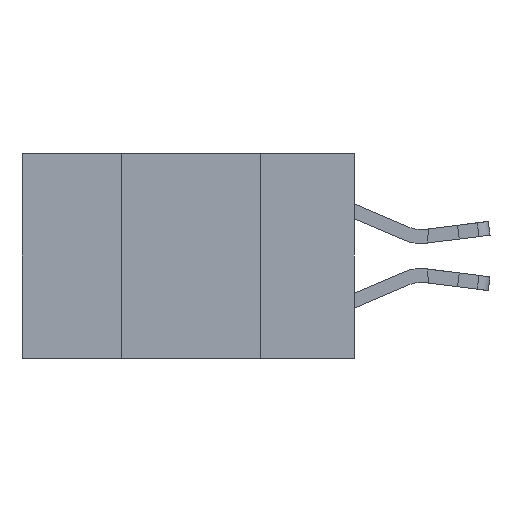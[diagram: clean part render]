
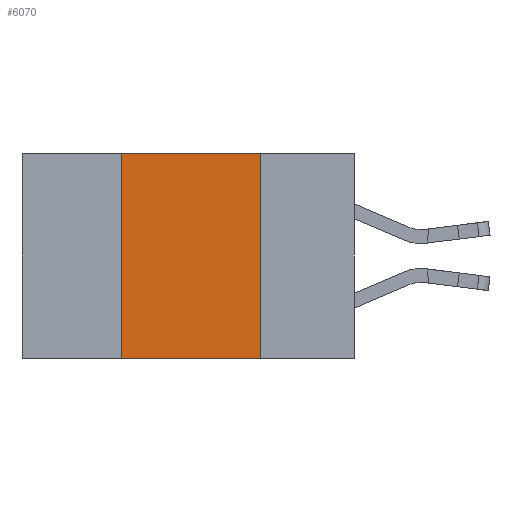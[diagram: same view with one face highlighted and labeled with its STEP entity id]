
A CAD part, left-side view. The second image highlights one B-rep face of the part: STEP entity #6070.
In plain terms, the highlighted planar face has unit normal (-1, 0, 0).
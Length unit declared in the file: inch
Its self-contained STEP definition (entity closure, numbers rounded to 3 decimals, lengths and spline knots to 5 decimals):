
#163 = CARTESIAN_POINT ( 'NONE',  ( 0., 0.17, 0. ) ) ;
#285 = LINE ( 'NONE', #12719, #1492 ) ;
#478 = EDGE_CURVE ( 'NONE', #17541, #1094, #5635, .T. ) ;
#940 = ORIENTED_EDGE ( 'NONE', *, *, #6986, .T. ) ;
#1094 = VERTEX_POINT ( 'NONE', #5809 ) ;
#1492 = VECTOR ( 'NONE', #6743, 39.37008 ) ;
#2147 = PLANE ( 'NONE',  #19913 ) ;
#2264 = ORIENTED_EDGE ( 'NONE', *, *, #478, .F. ) ;
#2501 = DIRECTION ( 'NONE',  ( 0., 0., -1. ) ) ;
#3178 = VECTOR ( 'NONE', #17279, 39.37008 ) ;
#5108 = ORIENTED_EDGE ( 'NONE', *, *, #9924, .F. ) ;
#5505 = CARTESIAN_POINT ( 'NONE',  ( 0., 0.42, 0. ) ) ;
#5540 = CARTESIAN_POINT ( 'NONE',  ( 0., 0.17, -0.37 ) ) ;
#5635 = LINE ( 'NONE', #5540, #11977 ) ;
#5809 = CARTESIAN_POINT ( 'NONE',  ( 0., 0.17, -0.37 ) ) ;
#5866 = DIRECTION ( 'NONE',  ( 0., 0., 1. ) ) ;
#6070 = ADVANCED_FACE ( 'NONE', ( #17820 ), #2147, .F. ) ;
#6140 = EDGE_CURVE ( 'NONE', #19836, #14645, #8601, .T. ) ;
#6457 = CARTESIAN_POINT ( 'NONE',  ( 0., 0.6, 0. ) ) ;
#6743 = DIRECTION ( 'NONE',  ( 0., -1., 0. ) ) ;
#6807 = EDGE_LOOP ( 'NONE', ( #2264, #5108, #13719, #940 ) ) ;
#6890 = CARTESIAN_POINT ( 'NONE',  ( 0., 0.6, 0. ) ) ;
#6986 = EDGE_CURVE ( 'NONE', #19836, #1094, #285, .T. ) ;
#7192 = CARTESIAN_POINT ( 'NONE',  ( 0., 0.42, -0.37 ) ) ;
#7610 = VECTOR ( 'NONE', #5866, 39.37008 ) ;
#8601 = LINE ( 'NONE', #7192, #7610 ) ;
#8812 = CARTESIAN_POINT ( 'NONE',  ( 0., 0.42, -0.37 ) ) ;
#9924 = EDGE_CURVE ( 'NONE', #14645, #17541, #14132, .T. ) ;
#11977 = VECTOR ( 'NONE', #2501, 39.37008 ) ;
#12719 = CARTESIAN_POINT ( 'NONE',  ( 0., 0.6, -0.37 ) ) ;
#13719 = ORIENTED_EDGE ( 'NONE', *, *, #6140, .F. ) ;
#14132 = LINE ( 'NONE', #6457, #3178 ) ;
#14645 = VERTEX_POINT ( 'NONE', #5505 ) ;
#16199 = DIRECTION ( 'NONE',  ( 0., 0., -1. ) ) ;
#17279 = DIRECTION ( 'NONE',  ( 0., -1., 0. ) ) ;
#17541 = VERTEX_POINT ( 'NONE', #163 ) ;
#17619 = DIRECTION ( 'NONE',  ( 1., 0., 0. ) ) ;
#17820 = FACE_OUTER_BOUND ( 'NONE', #6807, .T. ) ;
#19836 = VERTEX_POINT ( 'NONE', #8812 ) ;
#19913 = AXIS2_PLACEMENT_3D ( 'NONE', #6890, #17619, #16199 ) ;
